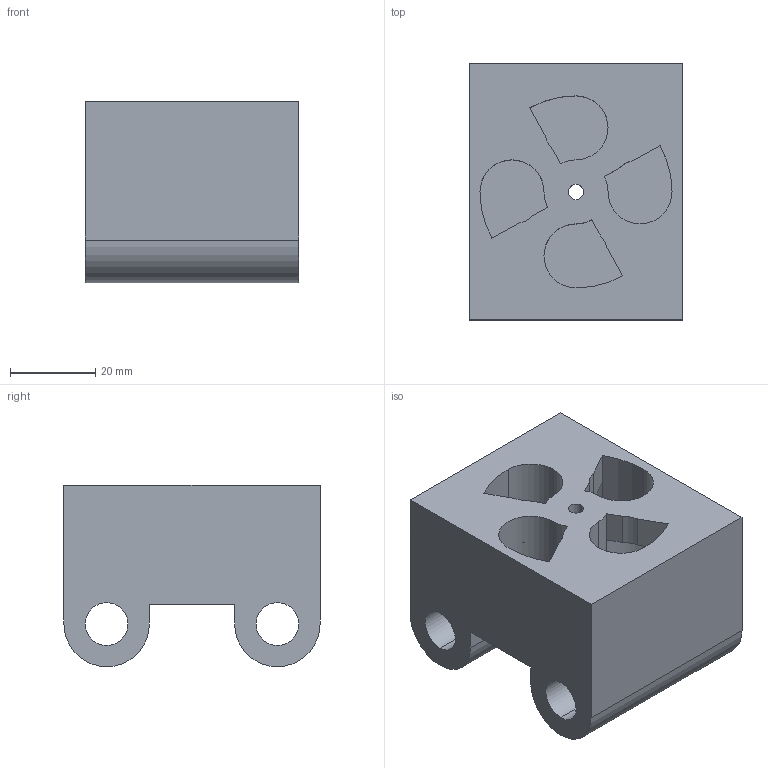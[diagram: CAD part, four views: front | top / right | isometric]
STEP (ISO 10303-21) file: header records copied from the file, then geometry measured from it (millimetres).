
FILE_DESCRIPTION (( 'STEP AP203' ), '1' );
FILE_NAME ('Hammer Body.STEP', '2013-08-28T12:50:25', ( '' ), ( '' ), 'SwSTEP 2.0', 'SolidWorks 2013', '' );
FILE_SCHEMA (( 'CONFIG_CONTROL_DESIGN' ));
Length unit declared in the file: millimetre
Products named in the file (1): Hammer Body
Bounding box: 50 x 60 x 42.5 mm (x, y, z)
Volume: 85607.1 mm3; surface area: 22523.9 mm2
Topology: 1 solids, 1 shells, 62 faces, 155 edges, 100 vertices
Faces by surface type: cylinder 35, plane 25, torus 2
Entity records: 1964 total; most frequent: DIRECTION 355, CARTESIAN_POINT 318, ORIENTED_EDGE 310, EDGE_CURVE 155, AXIS2_PLACEMENT_3D 137, VERTEX_POINT 100, VECTOR 81, LINE 81
